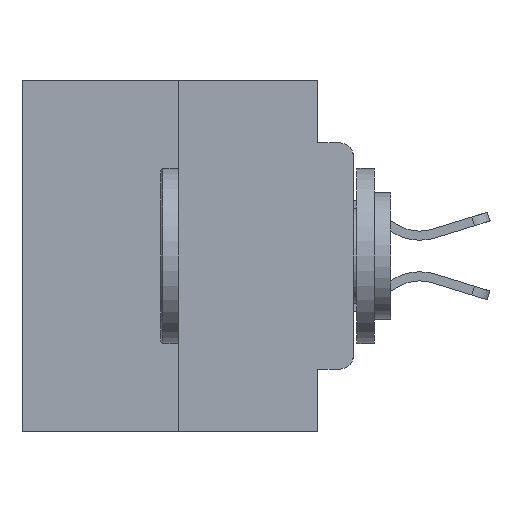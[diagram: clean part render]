
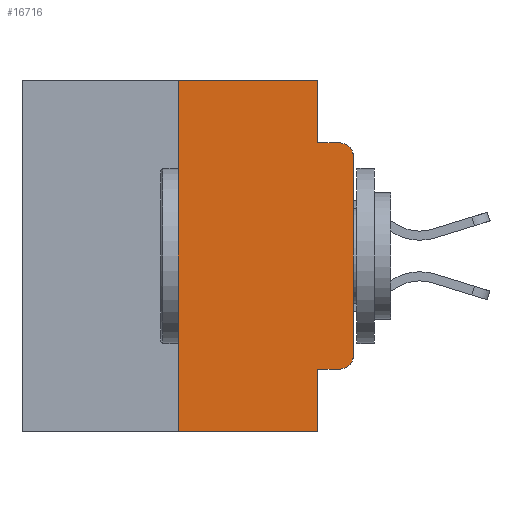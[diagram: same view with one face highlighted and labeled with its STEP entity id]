
A CAD part, left-side view. The second image highlights one B-rep face of the part: STEP entity #16716.
In plain terms, the highlighted planar face has unit normal (-1, 0, 0).
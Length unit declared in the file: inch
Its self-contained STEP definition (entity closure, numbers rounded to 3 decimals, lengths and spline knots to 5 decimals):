
#141 = EDGE_CURVE ( 'NONE', #18751, #15221, #8790, .T. ) ;
#266 = CARTESIAN_POINT ( 'NONE',  ( 0., 0.473, 0. ) ) ;
#1277 = CIRCLE ( 'NONE', #7063, 0.02 ) ;
#1821 = VERTEX_POINT ( 'NONE', #9065 ) ;
#1988 = VECTOR ( 'NONE', #5748, 39.37008 ) ;
#2344 = ORIENTED_EDGE ( 'NONE', *, *, #12870, .T. ) ;
#2582 = VECTOR ( 'NONE', #11365, 39.37008 ) ;
#2687 = LINE ( 'NONE', #3553, #1988 ) ;
#3051 = ORIENTED_EDGE ( 'NONE', *, *, #27496, .T. ) ;
#3553 = CARTESIAN_POINT ( 'NONE',  ( 0., 0.051, -0.4115 ) ) ;
#3728 = CARTESIAN_POINT ( 'NONE',  ( 0., 0.051, -0.4115 ) ) ;
#4110 = LINE ( 'NONE', #14209, #15590 ) ;
#4119 = ORIENTED_EDGE ( 'NONE', *, *, #141, .F. ) ;
#4141 = DIRECTION ( 'NONE',  ( 0., -1., 0. ) ) ;
#4164 = EDGE_CURVE ( 'NONE', #10605, #1821, #17044, .T. ) ;
#4838 = CARTESIAN_POINT ( 'NONE',  ( 0., 0.25, 0. ) ) ;
#4875 = VECTOR ( 'NONE', #4141, 39.37008 ) ;
#4974 = LINE ( 'NONE', #21104, #22077 ) ;
#5037 = VERTEX_POINT ( 'NONE', #24340 ) ;
#5748 = DIRECTION ( 'NONE',  ( 0., -1., 0. ) ) ;
#6085 = DIRECTION ( 'NONE',  ( 0., 0., 1. ) ) ;
#6154 = DIRECTION ( 'NONE',  ( -1., 0., 0. ) ) ;
#6159 = EDGE_CURVE ( 'NONE', #18751, #22487, #2687, .T. ) ;
#6839 = CARTESIAN_POINT ( 'NONE',  ( 0., 0.051, 0. ) ) ;
#7063 = AXIS2_PLACEMENT_3D ( 'NONE', #7100, #22058, #9255 ) ;
#7081 = CARTESIAN_POINT ( 'NONE',  ( 0., 0.02, -0.4115 ) ) ;
#7100 = CARTESIAN_POINT ( 'NONE',  ( 0., 0.02, -0.3915 ) ) ;
#8790 = LINE ( 'NONE', #6839, #25715 ) ;
#9065 = CARTESIAN_POINT ( 'NONE',  ( 0., 0.02, -0.0885 ) ) ;
#9255 = DIRECTION ( 'NONE',  ( 0., 0., -1. ) ) ;
#9598 = VERTEX_POINT ( 'NONE', #15680 ) ;
#9909 = VECTOR ( 'NONE', #20405, 39.37008 ) ;
#10197 = ORIENTED_EDGE ( 'NONE', *, *, #17350, .F. ) ;
#10605 = VERTEX_POINT ( 'NONE', #17064 ) ;
#10808 = EDGE_LOOP ( 'NONE', ( #2344, #3051, #14591, #20925, #10197, #24821, #14264, #4119, #21265, #27408 ) ) ;
#10851 = LINE ( 'NONE', #14089, #21553 ) ;
#11339 = PLANE ( 'NONE',  #22419 ) ;
#11365 = DIRECTION ( 'NONE',  ( 0., 0., 1. ) ) ;
#11960 = EDGE_CURVE ( 'NONE', #22085, #10605, #20654, .T. ) ;
#12870 = EDGE_CURVE ( 'NONE', #23674, #5037, #4974, .T. ) ;
#13517 = DIRECTION ( 'NONE',  ( 0., 0., -1. ) ) ;
#14089 = CARTESIAN_POINT ( 'NONE',  ( 0., 0.473, -0.5 ) ) ;
#14209 = CARTESIAN_POINT ( 'NONE',  ( 0., 0.473, 0. ) ) ;
#14264 = ORIENTED_EDGE ( 'NONE', *, *, #20195, .T. ) ;
#14591 = ORIENTED_EDGE ( 'NONE', *, *, #4164, .F. ) ;
#15221 = VERTEX_POINT ( 'NONE', #23599 ) ;
#15590 = VECTOR ( 'NONE', #20641, 39.37008 ) ;
#15680 = CARTESIAN_POINT ( 'NONE',  ( 0., 0.25, -0.5 ) ) ;
#16716 = ADVANCED_FACE ( 'NONE', ( #25167 ), #11339, .F. ) ;
#17044 = LINE ( 'NONE', #21239, #4875 ) ;
#17064 = CARTESIAN_POINT ( 'NONE',  ( 0., 0.051, -0.0885 ) ) ;
#17350 = EDGE_CURVE ( 'NONE', #26311, #22085, #4110, .T. ) ;
#17699 = CARTESIAN_POINT ( 'NONE',  ( 0., 0., -0.3915 ) ) ;
#18366 = CARTESIAN_POINT ( 'NONE',  ( 0., 0.051, 0. ) ) ;
#18751 = VERTEX_POINT ( 'NONE', #3728 ) ;
#19043 = CARTESIAN_POINT ( 'NONE',  ( 0., 0.02, -0.1085 ) ) ;
#19142 = EDGE_CURVE ( 'NONE', #9598, #26311, #19825, .T. ) ;
#19671 = EDGE_CURVE ( 'NONE', #22487, #23674, #1277, .T. ) ;
#19825 = LINE ( 'NONE', #4838, #2582 ) ;
#20195 = EDGE_CURVE ( 'NONE', #9598, #15221, #10851, .T. ) ;
#20405 = DIRECTION ( 'NONE',  ( 0., 0., -1. ) ) ;
#20641 = DIRECTION ( 'NONE',  ( 0., -1., 0. ) ) ;
#20654 = LINE ( 'NONE', #18366, #9909 ) ;
#20925 = ORIENTED_EDGE ( 'NONE', *, *, #11960, .F. ) ;
#21104 = CARTESIAN_POINT ( 'NONE',  ( 0., 0., 0. ) ) ;
#21163 = DIRECTION ( 'NONE',  ( 0., 0., -1. ) ) ;
#21239 = CARTESIAN_POINT ( 'NONE',  ( 0., 0.051, -0.0885 ) ) ;
#21265 = ORIENTED_EDGE ( 'NONE', *, *, #6159, .T. ) ;
#21553 = VECTOR ( 'NONE', #26673, 39.37008 ) ;
#21632 = CIRCLE ( 'NONE', #23934, 0.02 ) ;
#22058 = DIRECTION ( 'NONE',  ( -1., 0., 0. ) ) ;
#22077 = VECTOR ( 'NONE', #6085, 39.37008 ) ;
#22085 = VERTEX_POINT ( 'NONE', #24799 ) ;
#22419 = AXIS2_PLACEMENT_3D ( 'NONE', #266, #26113, #13517 ) ;
#22487 = VERTEX_POINT ( 'NONE', #7081 ) ;
#23599 = CARTESIAN_POINT ( 'NONE',  ( 0., 0.051, -0.5 ) ) ;
#23674 = VERTEX_POINT ( 'NONE', #17699 ) ;
#23934 = AXIS2_PLACEMENT_3D ( 'NONE', #19043, #6154, #21163 ) ;
#24340 = CARTESIAN_POINT ( 'NONE',  ( 0., 0., -0.1085 ) ) ;
#24671 = DIRECTION ( 'NONE',  ( 0., 0., -1. ) ) ;
#24799 = CARTESIAN_POINT ( 'NONE',  ( 0., 0.051, 0. ) ) ;
#24821 = ORIENTED_EDGE ( 'NONE', *, *, #19142, .F. ) ;
#25167 = FACE_OUTER_BOUND ( 'NONE', #10808, .T. ) ;
#25715 = VECTOR ( 'NONE', #24671, 39.37008 ) ;
#25730 = CARTESIAN_POINT ( 'NONE',  ( 0., 0.25, 0. ) ) ;
#26113 = DIRECTION ( 'NONE',  ( 1., 0., 0. ) ) ;
#26311 = VERTEX_POINT ( 'NONE', #25730 ) ;
#26673 = DIRECTION ( 'NONE',  ( 0., -1., 0. ) ) ;
#27408 = ORIENTED_EDGE ( 'NONE', *, *, #19671, .T. ) ;
#27496 = EDGE_CURVE ( 'NONE', #5037, #1821, #21632, .T. ) ;
